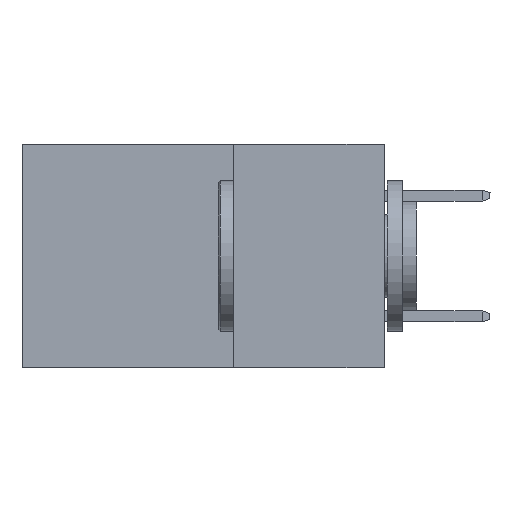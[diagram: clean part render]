
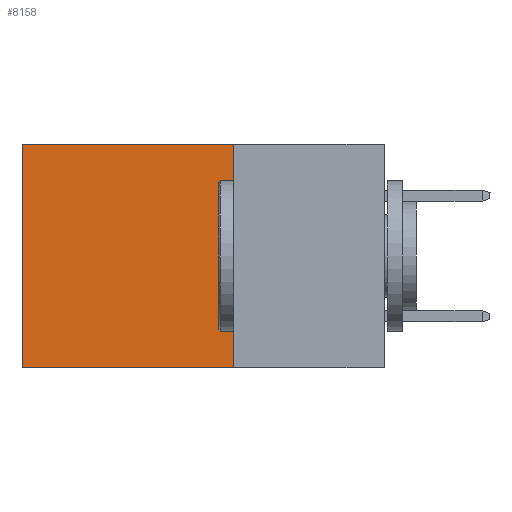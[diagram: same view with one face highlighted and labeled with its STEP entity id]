
A CAD part, left-side view. The second image highlights one B-rep face of the part: STEP entity #8158.
In plain terms, the highlighted planar face has unit normal (-1, 0, 0).
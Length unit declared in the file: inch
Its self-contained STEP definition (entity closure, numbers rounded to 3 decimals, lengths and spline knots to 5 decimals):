
#387 = DIRECTION ( 'NONE',  ( 1., 0., 0. ) ) ;
#425 = VECTOR ( 'NONE', #14581, 39.37008 ) ;
#580 = VECTOR ( 'NONE', #11233, 39.37008 ) ;
#1038 = CARTESIAN_POINT ( 'NONE',  ( 0.298, 0.25, 0. ) ) ;
#1276 = ORIENTED_EDGE ( 'NONE', *, *, #1739, .T. ) ;
#1739 = EDGE_CURVE ( 'NONE', #2804, #3156, #15800, .T. ) ;
#2268 = FACE_OUTER_BOUND ( 'NONE', #14163, .T. ) ;
#2444 = VERTEX_POINT ( 'NONE', #5163 ) ;
#2608 = EDGE_CURVE ( 'NONE', #3156, #2444, #12315, .T. ) ;
#2804 = VERTEX_POINT ( 'NONE', #1038 ) ;
#3156 = VERTEX_POINT ( 'NONE', #17119 ) ;
#4131 = EDGE_CURVE ( 'NONE', #2804, #11688, #9379, .T. ) ;
#4677 = PLANE ( 'NONE',  #8535 ) ;
#5163 = CARTESIAN_POINT ( 'NONE',  ( 0.298, 0.6, -0.37 ) ) ;
#6991 = VECTOR ( 'NONE', #16948, 39.37008 ) ;
#8158 = ADVANCED_FACE ( 'NONE', ( #2268 ), #4677, .F. ) ;
#8535 = AXIS2_PLACEMENT_3D ( 'NONE', #9223, #387, #10775 ) ;
#8755 = DIRECTION ( 'NONE',  ( 0., 1., 0. ) ) ;
#9172 = CARTESIAN_POINT ( 'NONE',  ( 0.298, 0.25, 0. ) ) ;
#9223 = CARTESIAN_POINT ( 'NONE',  ( 0.298, 0.25, 0. ) ) ;
#9379 = LINE ( 'NONE', #11367, #580 ) ;
#10775 = DIRECTION ( 'NONE',  ( 0., 0., -1. ) ) ;
#11233 = DIRECTION ( 'NONE',  ( 0., 0., -1. ) ) ;
#11367 = CARTESIAN_POINT ( 'NONE',  ( 0.298, 0.25, 0. ) ) ;
#11520 = CARTESIAN_POINT ( 'NONE',  ( 0.298, 0.6, 0. ) ) ;
#11688 = VERTEX_POINT ( 'NONE', #17239 ) ;
#11902 = VECTOR ( 'NONE', #8755, 39.37008 ) ;
#11967 = ORIENTED_EDGE ( 'NONE', *, *, #4131, .F. ) ;
#12315 = LINE ( 'NONE', #11520, #425 ) ;
#13032 = ORIENTED_EDGE ( 'NONE', *, *, #18552, .F. ) ;
#14163 = EDGE_LOOP ( 'NONE', ( #15208, #13032, #11967, #1276 ) ) ;
#14581 = DIRECTION ( 'NONE',  ( 0., 0., -1. ) ) ;
#15016 = LINE ( 'NONE', #15528, #6991 ) ;
#15208 = ORIENTED_EDGE ( 'NONE', *, *, #2608, .T. ) ;
#15528 = CARTESIAN_POINT ( 'NONE',  ( 0.298, 0.25, -0.37 ) ) ;
#15800 = LINE ( 'NONE', #9172, #11902 ) ;
#16948 = DIRECTION ( 'NONE',  ( 0., 1., 0. ) ) ;
#17119 = CARTESIAN_POINT ( 'NONE',  ( 0.298, 0.6, 0. ) ) ;
#17239 = CARTESIAN_POINT ( 'NONE',  ( 0.298, 0.25, -0.37 ) ) ;
#18552 = EDGE_CURVE ( 'NONE', #11688, #2444, #15016, .T. ) ;
